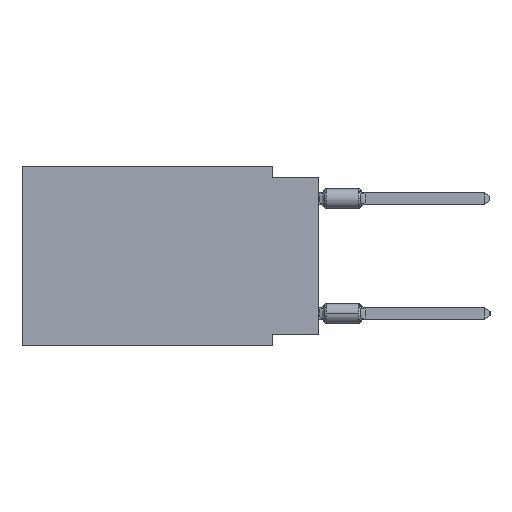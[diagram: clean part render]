
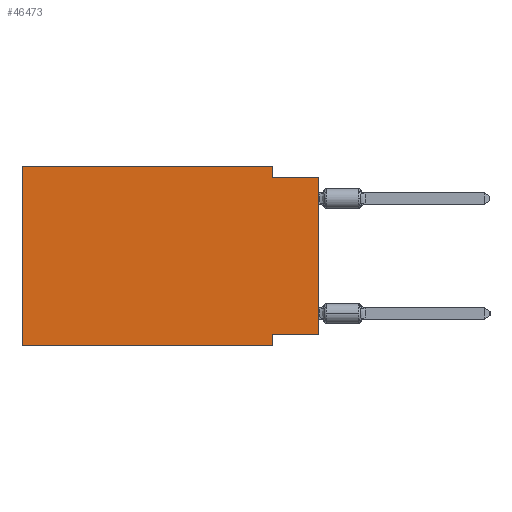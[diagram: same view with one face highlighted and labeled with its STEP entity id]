
A CAD part, left-side view. The second image highlights one B-rep face of the part: STEP entity #46473.
In plain terms, the highlighted planar face has unit normal (-1, 0, 0).
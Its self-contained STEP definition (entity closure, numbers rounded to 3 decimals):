
#1341 = ORIENTED_EDGE ( 'NONE', *, *, #40041, .F. ) ;
#1995 = ORIENTED_EDGE ( 'NONE', *, *, #13266, .T. ) ;
#2100 = VERTEX_POINT ( 'NONE', #40595 ) ;
#2981 = DIRECTION ( 'NONE',  ( 0., 0., -1. ) ) ;
#3246 = VECTOR ( 'NONE', #63276, 1000. ) ;
#6021 = CARTESIAN_POINT ( 'NONE',  ( 0., 0., 0. ) ) ;
#6244 = VECTOR ( 'NONE', #50346, 1000. ) ;
#7186 = ORIENTED_EDGE ( 'NONE', *, *, #12742, .F. ) ;
#11368 = VECTOR ( 'NONE', #45012, 1000. ) ;
#11420 = VERTEX_POINT ( 'NONE', #48463 ) ;
#12365 = EDGE_CURVE ( 'NONE', #30114, #11420, #53877, .T. ) ;
#12490 = CARTESIAN_POINT ( 'NONE',  ( 0., 2.54, -9.906 ) ) ;
#12742 = EDGE_CURVE ( 'NONE', #48944, #31992, #32474, .T. ) ;
#13266 = EDGE_CURVE ( 'NONE', #2100, #31992, #29661, .T. ) ;
#15353 = VECTOR ( 'NONE', #17909, 1000. ) ;
#15448 = CARTESIAN_POINT ( 'NONE',  ( 0., 2.54, -0.635 ) ) ;
#17578 = CARTESIAN_POINT ( 'NONE',  ( 0., 2.54, 0. ) ) ;
#17712 = ORIENTED_EDGE ( 'NONE', *, *, #52797, .F. ) ;
#17909 = DIRECTION ( 'NONE',  ( 0., 0., -1. ) ) ;
#19535 = VECTOR ( 'NONE', #24583, 1000. ) ;
#21576 = VECTOR ( 'NONE', #55561, 1000. ) ;
#21915 = ORIENTED_EDGE ( 'NONE', *, *, #50805, .T. ) ;
#23301 = CARTESIAN_POINT ( 'NONE',  ( 0., 16.383, 0. ) ) ;
#24277 = CARTESIAN_POINT ( 'NONE',  ( 0., 16.383, 0. ) ) ;
#24583 = DIRECTION ( 'NONE',  ( 0., 0., 1. ) ) ;
#27139 = VERTEX_POINT ( 'NONE', #15448 ) ;
#28958 = DIRECTION ( 'NONE',  ( 0., 1., 0. ) ) ;
#29661 = LINE ( 'NONE', #60164, #6244 ) ;
#30114 = VERTEX_POINT ( 'NONE', #62901 ) ;
#31359 = CARTESIAN_POINT ( 'NONE',  ( 0., 0., -0.635 ) ) ;
#31992 = VERTEX_POINT ( 'NONE', #32835 ) ;
#32474 = LINE ( 'NONE', #12490, #53408 ) ;
#32835 = CARTESIAN_POINT ( 'NONE',  ( 0., 2.54, -9.906 ) ) ;
#36353 = CARTESIAN_POINT ( 'NONE',  ( 0., 0., -9.271 ) ) ;
#38815 = LINE ( 'NONE', #57604, #45024 ) ;
#40041 = EDGE_CURVE ( 'NONE', #11420, #27139, #62842, .T. ) ;
#40228 = EDGE_LOOP ( 'NONE', ( #21915, #61828, #1341, #54094, #17712, #1995, #7186, #61091 ) ) ;
#40595 = CARTESIAN_POINT ( 'NONE',  ( 0., 16.383, -9.906 ) ) ;
#42666 = FACE_OUTER_BOUND ( 'NONE', #40228, .T. ) ;
#42968 = LINE ( 'NONE', #58029, #3246 ) ;
#43005 = DIRECTION ( 'NONE',  ( 1., 0., 0. ) ) ;
#45012 = DIRECTION ( 'NONE',  ( 0., -1., 0. ) ) ;
#45024 = VECTOR ( 'NONE', #28958, 1000. ) ;
#45172 = CARTESIAN_POINT ( 'NONE',  ( 0., 2.54, -9.271 ) ) ;
#46473 = ADVANCED_FACE ( 'NONE', ( #42666 ), #62674, .F. ) ;
#48463 = CARTESIAN_POINT ( 'NONE',  ( 0., 2.54, 0. ) ) ;
#48944 = VERTEX_POINT ( 'NONE', #45172 ) ;
#49241 = LINE ( 'NONE', #24277, #19535 ) ;
#50346 = DIRECTION ( 'NONE',  ( 0., -1., 0. ) ) ;
#50805 = EDGE_CURVE ( 'NONE', #52826, #58666, #60810, .T. ) ;
#52797 = EDGE_CURVE ( 'NONE', #2100, #30114, #49241, .T. ) ;
#52826 = VERTEX_POINT ( 'NONE', #36353 ) ;
#53408 = VECTOR ( 'NONE', #2981, 1000. ) ;
#53877 = LINE ( 'NONE', #63718, #11368 ) ;
#54094 = ORIENTED_EDGE ( 'NONE', *, *, #12365, .F. ) ;
#55561 = DIRECTION ( 'NONE',  ( 0., 0., 1. ) ) ;
#57604 = CARTESIAN_POINT ( 'NONE',  ( 0., 0., -9.271 ) ) ;
#58029 = CARTESIAN_POINT ( 'NONE',  ( 0., 0., -0.635 ) ) ;
#58412 = DIRECTION ( 'NONE',  ( 0., 0., -1. ) ) ;
#58666 = VERTEX_POINT ( 'NONE', #31359 ) ;
#60164 = CARTESIAN_POINT ( 'NONE',  ( 0., 16.383, -9.906 ) ) ;
#60541 = EDGE_CURVE ( 'NONE', #52826, #48944, #38815, .T. ) ;
#60810 = LINE ( 'NONE', #6021, #21576 ) ;
#61091 = ORIENTED_EDGE ( 'NONE', *, *, #60541, .F. ) ;
#61828 = ORIENTED_EDGE ( 'NONE', *, *, #64028, .F. ) ;
#62674 = PLANE ( 'NONE',  #63335 ) ;
#62842 = LINE ( 'NONE', #17578, #15353 ) ;
#62901 = CARTESIAN_POINT ( 'NONE',  ( 0., 16.383, 0. ) ) ;
#63276 = DIRECTION ( 'NONE',  ( 0., -1., 0. ) ) ;
#63335 = AXIS2_PLACEMENT_3D ( 'NONE', #23301, #43005, #58412 ) ;
#63718 = CARTESIAN_POINT ( 'NONE',  ( 0., 16.383, 0. ) ) ;
#64028 = EDGE_CURVE ( 'NONE', #27139, #58666, #42968, .T. ) ;
